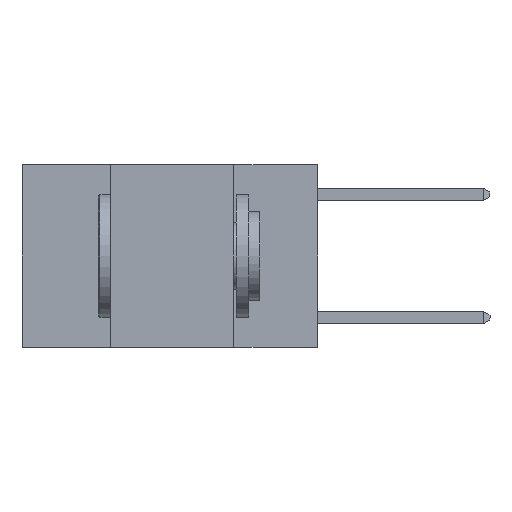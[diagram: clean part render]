
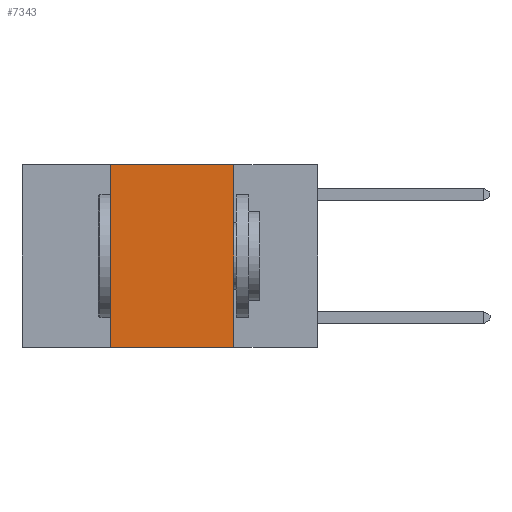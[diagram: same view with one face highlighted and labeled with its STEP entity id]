
A CAD part, left-side view. The second image highlights one B-rep face of the part: STEP entity #7343.
In plain terms, the highlighted planar face has unit normal (-1, 0, 0).
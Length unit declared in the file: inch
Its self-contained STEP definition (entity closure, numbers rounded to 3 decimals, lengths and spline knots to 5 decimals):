
#864 = VECTOR ( 'NONE', #10778, 39.37008 ) ;
#1092 = VECTOR ( 'NONE', #11268, 39.37008 ) ;
#1100 = CARTESIAN_POINT ( 'NONE',  ( 0., 0.42, 0. ) ) ;
#1302 = ORIENTED_EDGE ( 'NONE', *, *, #10352, .F. ) ;
#1305 = CARTESIAN_POINT ( 'NONE',  ( 0., 0.6, -0.37 ) ) ;
#1384 = LINE ( 'NONE', #1305, #10938 ) ;
#1622 = VECTOR ( 'NONE', #4799, 39.37008 ) ;
#1708 = VERTEX_POINT ( 'NONE', #2867 ) ;
#2758 = DIRECTION ( 'NONE',  ( 1., 0., 0. ) ) ;
#2867 = CARTESIAN_POINT ( 'NONE',  ( 0., 0.42, -0.37 ) ) ;
#2890 = VERTEX_POINT ( 'NONE', #10878 ) ;
#3285 = CARTESIAN_POINT ( 'NONE',  ( 0., 0.42, 0. ) ) ;
#3447 = FACE_OUTER_BOUND ( 'NONE', #10050, .T. ) ;
#3702 = VERTEX_POINT ( 'NONE', #11240 ) ;
#3784 = AXIS2_PLACEMENT_3D ( 'NONE', #5505, #2758, #9319 ) ;
#3873 = EDGE_CURVE ( 'NONE', #1708, #3702, #1384, .T. ) ;
#4569 = EDGE_CURVE ( 'NONE', #2890, #3702, #8521, .T. ) ;
#4799 = DIRECTION ( 'NONE',  ( 0., -1., 0. ) ) ;
#4841 = CARTESIAN_POINT ( 'NONE',  ( 0., 0.6, 0. ) ) ;
#5113 = EDGE_CURVE ( 'NONE', #5500, #2890, #11460, .T. ) ;
#5500 = VERTEX_POINT ( 'NONE', #1100 ) ;
#5505 = CARTESIAN_POINT ( 'NONE',  ( 0., 0.6, 0. ) ) ;
#7343 = ADVANCED_FACE ( 'NONE', ( #3447 ), #8417, .F. ) ;
#8288 = LINE ( 'NONE', #3285, #864 ) ;
#8417 = PLANE ( 'NONE',  #3784 ) ;
#8440 = ORIENTED_EDGE ( 'NONE', *, *, #4569, .F. ) ;
#8521 = LINE ( 'NONE', #10363, #1092 ) ;
#8729 = ORIENTED_EDGE ( 'NONE', *, *, #3873, .T. ) ;
#8745 = DIRECTION ( 'NONE',  ( 0., -1., 0. ) ) ;
#9319 = DIRECTION ( 'NONE',  ( 0., 0., -1. ) ) ;
#10050 = EDGE_LOOP ( 'NONE', ( #8440, #10856, #1302, #8729 ) ) ;
#10352 = EDGE_CURVE ( 'NONE', #1708, #5500, #8288, .T. ) ;
#10363 = CARTESIAN_POINT ( 'NONE',  ( 0., 0.17, 0. ) ) ;
#10778 = DIRECTION ( 'NONE',  ( 0., 0., 1. ) ) ;
#10856 = ORIENTED_EDGE ( 'NONE', *, *, #5113, .F. ) ;
#10878 = CARTESIAN_POINT ( 'NONE',  ( 0., 0.17, 0. ) ) ;
#10938 = VECTOR ( 'NONE', #8745, 39.37008 ) ;
#11240 = CARTESIAN_POINT ( 'NONE',  ( 0., 0.17, -0.37 ) ) ;
#11268 = DIRECTION ( 'NONE',  ( 0., 0., -1. ) ) ;
#11460 = LINE ( 'NONE', #4841, #1622 ) ;
